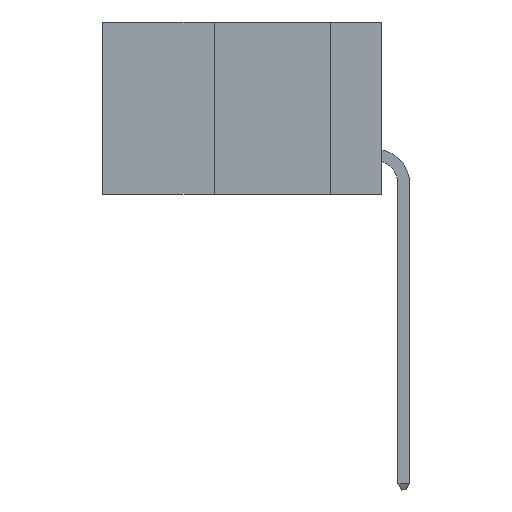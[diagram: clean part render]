
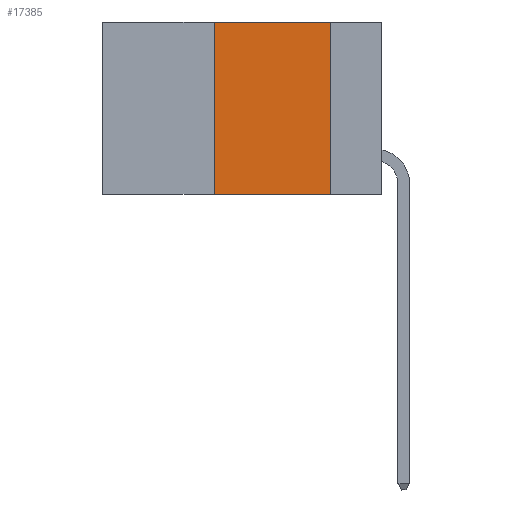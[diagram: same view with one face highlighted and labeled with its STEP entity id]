
A CAD part, left-side view. The second image highlights one B-rep face of the part: STEP entity #17385.
In plain terms, the highlighted planar face has unit normal (-1, 0, 0).
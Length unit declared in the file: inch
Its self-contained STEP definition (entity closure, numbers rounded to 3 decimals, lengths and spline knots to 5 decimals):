
#753 = EDGE_CURVE ( 'NONE', #21103, #4446, #24348, .T. ) ;
#2390 = ORIENTED_EDGE ( 'NONE', *, *, #753, .F. ) ;
#2619 = VECTOR ( 'NONE', #8011, 39.37008 ) ;
#4446 = VERTEX_POINT ( 'NONE', #12553 ) ;
#5280 = AXIS2_PLACEMENT_3D ( 'NONE', #13324, #15075, #9321 ) ;
#5683 = CARTESIAN_POINT ( 'NONE',  ( 0., 0.11, 0. ) ) ;
#5990 = ORIENTED_EDGE ( 'NONE', *, *, #7428, .T. ) ;
#7428 = EDGE_CURVE ( 'NONE', #25300, #4446, #24721, .T. ) ;
#8011 = DIRECTION ( 'NONE',  ( 0., -1., 0. ) ) ;
#8699 = DIRECTION ( 'NONE',  ( 0., 0., -1. ) ) ;
#9321 = DIRECTION ( 'NONE',  ( 0., 0., -1. ) ) ;
#9376 = CARTESIAN_POINT ( 'NONE',  ( 0., 0.6, 0. ) ) ;
#9703 = ORIENTED_EDGE ( 'NONE', *, *, #14102, .F. ) ;
#9810 = EDGE_CURVE ( 'NONE', #20636, #21103, #19968, .T. ) ;
#10368 = CARTESIAN_POINT ( 'NONE',  ( 0., 0.36, 0. ) ) ;
#10555 = EDGE_LOOP ( 'NONE', ( #2390, #22630, #9703, #5990 ) ) ;
#12553 = CARTESIAN_POINT ( 'NONE',  ( 0., 0.11, -0.37 ) ) ;
#13324 = CARTESIAN_POINT ( 'NONE',  ( 0., 0.6, 0. ) ) ;
#13810 = DIRECTION ( 'NONE',  ( 0., 0., 1. ) ) ;
#14102 = EDGE_CURVE ( 'NONE', #25300, #20636, #19827, .T. ) ;
#14167 = CARTESIAN_POINT ( 'NONE',  ( 0., 0.11, 0. ) ) ;
#14206 = VECTOR ( 'NONE', #14673, 39.37008 ) ;
#14673 = DIRECTION ( 'NONE',  ( 0., -1., 0. ) ) ;
#15075 = DIRECTION ( 'NONE',  ( 1., 0., 0. ) ) ;
#16931 = VECTOR ( 'NONE', #8699, 39.37008 ) ;
#17108 = FACE_OUTER_BOUND ( 'NONE', #10555, .T. ) ;
#17213 = PLANE ( 'NONE',  #5280 ) ;
#17385 = ADVANCED_FACE ( 'NONE', ( #17108 ), #17213, .F. ) ;
#17950 = VECTOR ( 'NONE', #13810, 39.37008 ) ;
#18381 = CARTESIAN_POINT ( 'NONE',  ( 0., 0.6, -0.37 ) ) ;
#19401 = CARTESIAN_POINT ( 'NONE',  ( 0., 0.36, -0.37 ) ) ;
#19827 = LINE ( 'NONE', #23645, #17950 ) ;
#19968 = LINE ( 'NONE', #9376, #2619 ) ;
#20636 = VERTEX_POINT ( 'NONE', #10368 ) ;
#21103 = VERTEX_POINT ( 'NONE', #5683 ) ;
#22630 = ORIENTED_EDGE ( 'NONE', *, *, #9810, .F. ) ;
#23645 = CARTESIAN_POINT ( 'NONE',  ( 0., 0.36, 0. ) ) ;
#24348 = LINE ( 'NONE', #14167, #16931 ) ;
#24721 = LINE ( 'NONE', #18381, #14206 ) ;
#25300 = VERTEX_POINT ( 'NONE', #19401 ) ;
